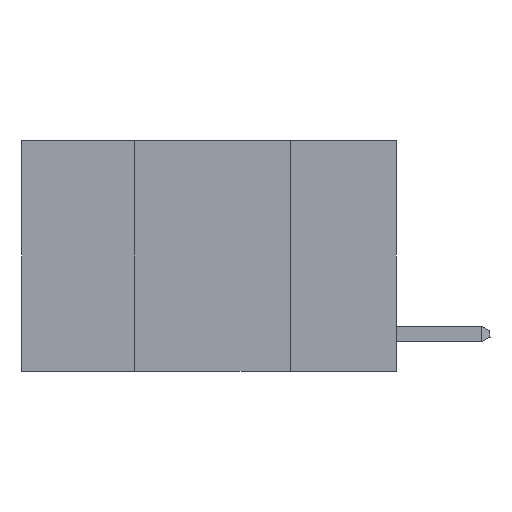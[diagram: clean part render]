
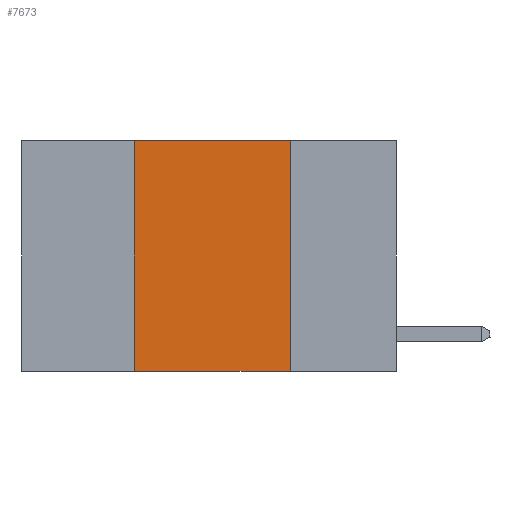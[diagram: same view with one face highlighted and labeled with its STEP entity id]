
A CAD part, left-side view. The second image highlights one B-rep face of the part: STEP entity #7673.
In plain terms, the highlighted planar face has unit normal (-1, 0, 0).
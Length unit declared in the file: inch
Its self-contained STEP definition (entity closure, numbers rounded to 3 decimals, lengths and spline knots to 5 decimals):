
#594 = EDGE_CURVE ( 'NONE', #11724, #8896, #20836, .T. ) ;
#966 = EDGE_CURVE ( 'NONE', #8896, #11920, #2670, .T. ) ;
#1754 = DIRECTION ( 'NONE',  ( 0., 0., 1. ) ) ;
#1813 = PLANE ( 'NONE',  #5089 ) ;
#1837 = EDGE_LOOP ( 'NONE', ( #13748, #6717, #8405, #4904 ) ) ;
#2670 = LINE ( 'NONE', #15646, #9975 ) ;
#3390 = VECTOR ( 'NONE', #1754, 39.37008 ) ;
#3613 = FACE_OUTER_BOUND ( 'NONE', #1837, .T. ) ;
#4040 = EDGE_CURVE ( 'NONE', #11724, #11336, #16416, .T. ) ;
#4885 = EDGE_CURVE ( 'NONE', #11920, #11336, #11246, .T. ) ;
#4904 = ORIENTED_EDGE ( 'NONE', *, *, #4040, .T. ) ;
#4919 = DIRECTION ( 'NONE',  ( 0., 0., -1. ) ) ;
#5089 = AXIS2_PLACEMENT_3D ( 'NONE', #9773, #11602, #4919 ) ;
#6717 = ORIENTED_EDGE ( 'NONE', *, *, #966, .F. ) ;
#6718 = CARTESIAN_POINT ( 'NONE',  ( 0., 0.42, -0.37 ) ) ;
#7458 = CARTESIAN_POINT ( 'NONE',  ( 0., 0.17, 0. ) ) ;
#7673 = ADVANCED_FACE ( 'NONE', ( #3613 ), #1813, .F. ) ;
#7905 = DIRECTION ( 'NONE',  ( 0., 0., -1. ) ) ;
#7984 = CARTESIAN_POINT ( 'NONE',  ( 0., 0.42, 0. ) ) ;
#8405 = ORIENTED_EDGE ( 'NONE', *, *, #594, .F. ) ;
#8896 = VERTEX_POINT ( 'NONE', #17911 ) ;
#9773 = CARTESIAN_POINT ( 'NONE',  ( 0., 0.6, 0. ) ) ;
#9975 = VECTOR ( 'NONE', #18796, 39.37008 ) ;
#11213 = CARTESIAN_POINT ( 'NONE',  ( 0., 0.6, -0.37 ) ) ;
#11246 = LINE ( 'NONE', #12874, #12312 ) ;
#11336 = VERTEX_POINT ( 'NONE', #13346 ) ;
#11602 = DIRECTION ( 'NONE',  ( 1., 0., 0. ) ) ;
#11724 = VERTEX_POINT ( 'NONE', #6718 ) ;
#11920 = VERTEX_POINT ( 'NONE', #7458 ) ;
#12312 = VECTOR ( 'NONE', #7905, 39.37008 ) ;
#12874 = CARTESIAN_POINT ( 'NONE',  ( 0., 0.17, 0. ) ) ;
#13346 = CARTESIAN_POINT ( 'NONE',  ( 0., 0.17, -0.37 ) ) ;
#13748 = ORIENTED_EDGE ( 'NONE', *, *, #4885, .F. ) ;
#14207 = VECTOR ( 'NONE', #19346, 39.37008 ) ;
#15646 = CARTESIAN_POINT ( 'NONE',  ( 0., 0.6, 0. ) ) ;
#16416 = LINE ( 'NONE', #11213, #14207 ) ;
#17911 = CARTESIAN_POINT ( 'NONE',  ( 0., 0.42, 0. ) ) ;
#18796 = DIRECTION ( 'NONE',  ( 0., -1., 0. ) ) ;
#19346 = DIRECTION ( 'NONE',  ( 0., -1., 0. ) ) ;
#20836 = LINE ( 'NONE', #7984, #3390 ) ;
